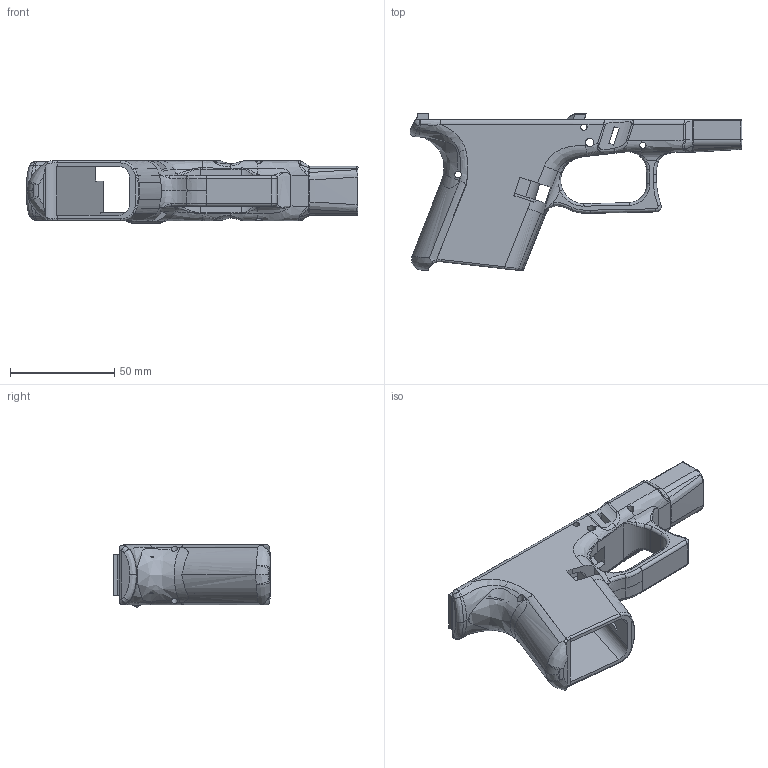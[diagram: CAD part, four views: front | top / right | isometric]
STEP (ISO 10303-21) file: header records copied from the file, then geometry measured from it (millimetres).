
FILE_DESCRIPTION(/* description */ (''),/* implementation_level */ '2;1');
FILE_NAME(/* name */ 'FMDA G26.2 V1.17 G5Spring Frame.stp',/* time_stamp */ '2021-05-04T15:33:32-05:00',/* author */ ('johne'),/* organization */ (''),/* preprocessor_version */ 'ST-DEVELOPER v18',/* originating_system */ 'Autodesk Inventor 2020',/* authorisation */ '');
FILE_SCHEMA (('AUTOMOTIVE_DESIGN { 1 0 10303 214 3 1 1 }'));
Products named in the file (1): FMDA G26.2 V1.16 G5Spring Frame
Bounding box: 159.33 x 75.32 x 29.84 mm (x, y, z)
Volume: 64006.1 mm3; surface area: 35679.3 mm2
Topology: 1 solids, 3 shells, 494 faces, 1483 edges, 967 vertices
Faces by surface type: bspline 198, plane 145, cylinder 105, torus 27, sphere 10, cone 9
Full cylindrical faces by diameter (mm): 2 x1, 3 x4, 3.2 x2, 3.81 x1, 4 x2
Entity records: 42297 total; most frequent: CARTESIAN_POINT 29752, ORIENTED_EDGE 2936, DIRECTION 2050, EDGE_CURVE 1468, VERTEX_POINT 959, AXIS2_PLACEMENT_3D 758, LINE 534, VECTOR 534
